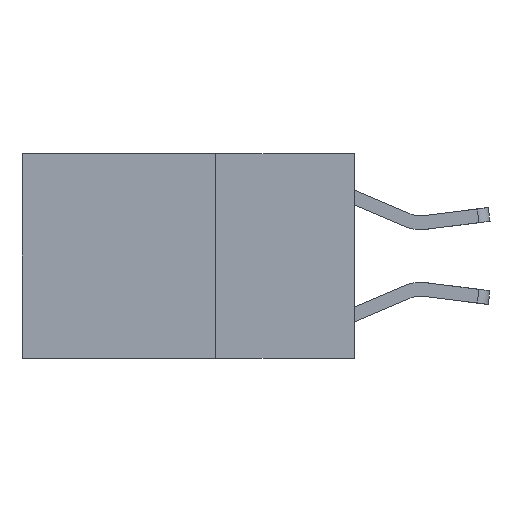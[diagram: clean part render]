
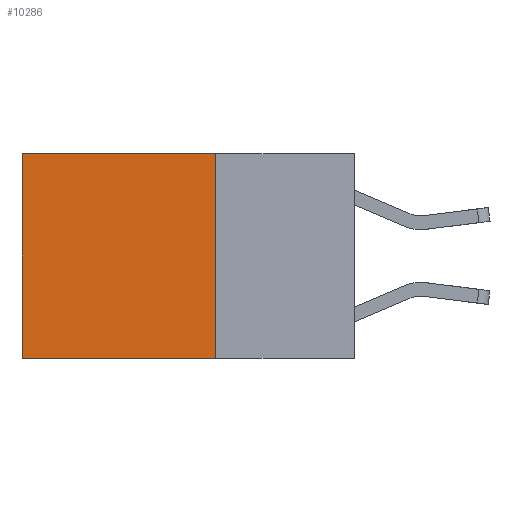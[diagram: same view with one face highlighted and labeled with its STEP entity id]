
A CAD part, left-side view. The second image highlights one B-rep face of the part: STEP entity #10286.
In plain terms, the highlighted planar face has unit normal (-1, 0, 0).
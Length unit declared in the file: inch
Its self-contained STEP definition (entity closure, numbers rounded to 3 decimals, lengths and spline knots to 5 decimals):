
#300 = AXIS2_PLACEMENT_3D ( 'NONE', #1012, #1200, #508 ) ;
#508 = DIRECTION ( 'NONE',  ( 0., 0., -1. ) ) ;
#1012 = CARTESIAN_POINT ( 'NONE',  ( 0.2625, 0.25, 0. ) ) ;
#1085 = ORIENTED_EDGE ( 'NONE', *, *, #2104, .T. ) ;
#1200 = DIRECTION ( 'NONE',  ( 1., 0., 0. ) ) ;
#1207 = EDGE_CURVE ( 'NONE', #5601, #2849, #10569, .T. ) ;
#1603 = ORIENTED_EDGE ( 'NONE', *, *, #1207, .T. ) ;
#1662 = DIRECTION ( 'NONE',  ( 0., 0., -1. ) ) ;
#2104 = EDGE_CURVE ( 'NONE', #2849, #9109, #2560, .T. ) ;
#2560 = LINE ( 'NONE', #5058, #6626 ) ;
#2849 = VERTEX_POINT ( 'NONE', #10526 ) ;
#3253 = DIRECTION ( 'NONE',  ( 0., 1., 0. ) ) ;
#3603 = CARTESIAN_POINT ( 'NONE',  ( 0.2625, 0.6, -0.37 ) ) ;
#3618 = LINE ( 'NONE', #4207, #6722 ) ;
#4207 = CARTESIAN_POINT ( 'NONE',  ( 0.2625, 0.25, 0. ) ) ;
#4390 = ORIENTED_EDGE ( 'NONE', *, *, #8789, .F. ) ;
#4621 = VECTOR ( 'NONE', #3253, 39.37008 ) ;
#4691 = CARTESIAN_POINT ( 'NONE',  ( 0.2625, 0.25, 0. ) ) ;
#4799 = ORIENTED_EDGE ( 'NONE', *, *, #7859, .F. ) ;
#5022 = CARTESIAN_POINT ( 'NONE',  ( 0.2625, 0.25, 0. ) ) ;
#5058 = CARTESIAN_POINT ( 'NONE',  ( 0.2625, 0.6, 0. ) ) ;
#5601 = VERTEX_POINT ( 'NONE', #4691 ) ;
#5840 = CARTESIAN_POINT ( 'NONE',  ( 0.2625, 0.25, -0.37 ) ) ;
#6626 = VECTOR ( 'NONE', #7516, 39.37008 ) ;
#6722 = VECTOR ( 'NONE', #1662, 39.37008 ) ;
#6780 = DIRECTION ( 'NONE',  ( 0., 1., 0. ) ) ;
#6916 = VECTOR ( 'NONE', #6780, 39.37008 ) ;
#6950 = EDGE_LOOP ( 'NONE', ( #1085, #4390, #4799, #1603 ) ) ;
#7120 = LINE ( 'NONE', #5840, #4621 ) ;
#7516 = DIRECTION ( 'NONE',  ( 0., 0., -1. ) ) ;
#7708 = CARTESIAN_POINT ( 'NONE',  ( 0.2625, 0.25, -0.37 ) ) ;
#7728 = FACE_OUTER_BOUND ( 'NONE', #6950, .T. ) ;
#7859 = EDGE_CURVE ( 'NONE', #5601, #10413, #3618, .T. ) ;
#8789 = EDGE_CURVE ( 'NONE', #10413, #9109, #7120, .T. ) ;
#9109 = VERTEX_POINT ( 'NONE', #3603 ) ;
#9477 = PLANE ( 'NONE',  #300 ) ;
#10286 = ADVANCED_FACE ( 'NONE', ( #7728 ), #9477, .F. ) ;
#10413 = VERTEX_POINT ( 'NONE', #7708 ) ;
#10526 = CARTESIAN_POINT ( 'NONE',  ( 0.2625, 0.6, 0. ) ) ;
#10569 = LINE ( 'NONE', #5022, #6916 ) ;
